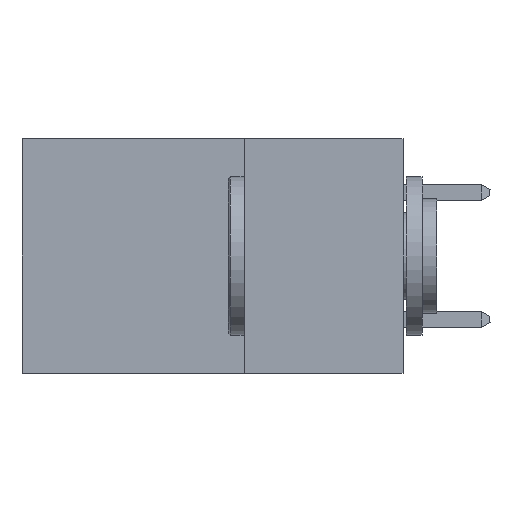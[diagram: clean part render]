
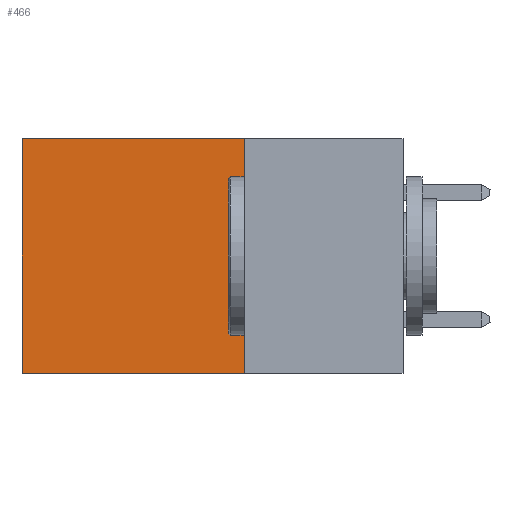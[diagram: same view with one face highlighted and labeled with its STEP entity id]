
A CAD part, left-side view. The second image highlights one B-rep face of the part: STEP entity #466.
In plain terms, the highlighted planar face has unit normal (-1, 0, 0).
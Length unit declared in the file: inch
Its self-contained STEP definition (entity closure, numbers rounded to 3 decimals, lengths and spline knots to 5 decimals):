
#466 = ADVANCED_FACE ( 'NONE', ( #12040 ), #34752, .F. ) ;
#628 = CARTESIAN_POINT ( 'NONE',  ( 0.2875, 0.6, -0.37 ) ) ;
#1238 = VERTEX_POINT ( 'NONE', #20636 ) ;
#3183 = ORIENTED_EDGE ( 'NONE', *, *, #10865, .T. ) ;
#3435 = DIRECTION ( 'NONE',  ( 0., 1., 0. ) ) ;
#3839 = VERTEX_POINT ( 'NONE', #628 ) ;
#4103 = EDGE_CURVE ( 'NONE', #10181, #1238, #16506, .T. ) ;
#5827 = VECTOR ( 'NONE', #20052, 39.37008 ) ;
#6177 = VERTEX_POINT ( 'NONE', #26889 ) ;
#9413 = LINE ( 'NONE', #34327, #30119 ) ;
#10181 = VERTEX_POINT ( 'NONE', #35151 ) ;
#10865 = EDGE_CURVE ( 'NONE', #6177, #3839, #36388, .T. ) ;
#12040 = FACE_OUTER_BOUND ( 'NONE', #12108, .T. ) ;
#12108 = EDGE_LOOP ( 'NONE', ( #3183, #27002, #36275, #16628 ) ) ;
#12275 = EDGE_CURVE ( 'NONE', #10181, #6177, #17320, .T. ) ;
#12385 = DIRECTION ( 'NONE',  ( 0., 0., -1. ) ) ;
#15658 = VECTOR ( 'NONE', #12385, 39.37008 ) ;
#16506 = LINE ( 'NONE', #34145, #5827 ) ;
#16628 = ORIENTED_EDGE ( 'NONE', *, *, #12275, .T. ) ;
#17320 = LINE ( 'NONE', #26822, #34320 ) ;
#17640 = EDGE_CURVE ( 'NONE', #1238, #3839, #9413, .T. ) ;
#18139 = DIRECTION ( 'NONE',  ( 1., 0., 0. ) ) ;
#18661 = CARTESIAN_POINT ( 'NONE',  ( 0.2875, 0.6, 0. ) ) ;
#20052 = DIRECTION ( 'NONE',  ( 0., 0., -1. ) ) ;
#20636 = CARTESIAN_POINT ( 'NONE',  ( 0.2875, 0.25, -0.37 ) ) ;
#23321 = AXIS2_PLACEMENT_3D ( 'NONE', #42103, #18139, #38663 ) ;
#26822 = CARTESIAN_POINT ( 'NONE',  ( 0.2875, 0.25, 0. ) ) ;
#26889 = CARTESIAN_POINT ( 'NONE',  ( 0.2875, 0.6, 0. ) ) ;
#27002 = ORIENTED_EDGE ( 'NONE', *, *, #17640, .F. ) ;
#30119 = VECTOR ( 'NONE', #3435, 39.37008 ) ;
#33774 = DIRECTION ( 'NONE',  ( 0., 1., 0. ) ) ;
#34145 = CARTESIAN_POINT ( 'NONE',  ( 0.2875, 0.25, 0. ) ) ;
#34320 = VECTOR ( 'NONE', #33774, 39.37008 ) ;
#34327 = CARTESIAN_POINT ( 'NONE',  ( 0.2875, 0.25, -0.37 ) ) ;
#34752 = PLANE ( 'NONE',  #23321 ) ;
#35151 = CARTESIAN_POINT ( 'NONE',  ( 0.2875, 0.25, 0. ) ) ;
#36275 = ORIENTED_EDGE ( 'NONE', *, *, #4103, .F. ) ;
#36388 = LINE ( 'NONE', #18661, #15658 ) ;
#38663 = DIRECTION ( 'NONE',  ( 0., 0., -1. ) ) ;
#42103 = CARTESIAN_POINT ( 'NONE',  ( 0.2875, 0.25, 0. ) ) ;
